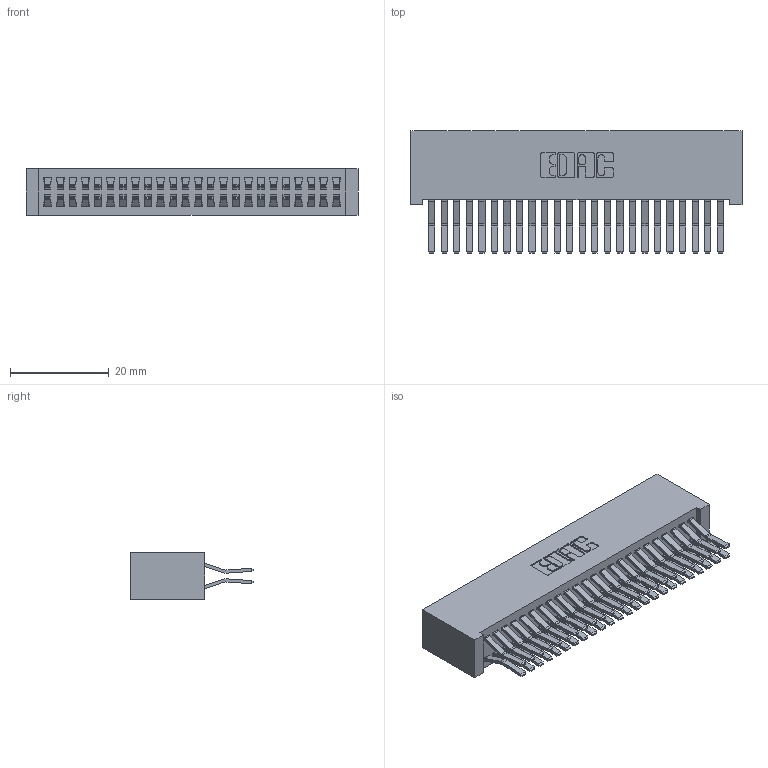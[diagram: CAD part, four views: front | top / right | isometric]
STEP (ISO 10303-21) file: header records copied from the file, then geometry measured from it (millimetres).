
FILE_DESCRIPTION (( 'STEP AP203' ), '1' );
FILE_NAME ('392-048-560-201.STEP', '2019-10-08T01:37:07', ( '' ), ( '' ), 'SwSTEP 2.0', 'SolidWorks 2016', '' );
FILE_SCHEMA (( 'CONFIG_CONTROL_DESIGN' ));
Length unit declared in the file: inch
Products named in the file (3): 342 Part_Lugless; 345-292-001_560 Tail; 392-048-560-201
Assembly tree (49 placements, depth 2):
  392-048-560-201
    342 Part_Lugless
    345-292-001_560 Tail  x48
Bounding box: 67.21 x 24.78 x 9.4 mm (x, y, z)
Volume: 6708.1 mm3; surface area: 11677.5 mm2
Topology: 49 solids, 49 shells, 2694 faces, 8003 edges, 5270 vertices
Faces by surface type: plane 1790, cylinder 904
Entity records: 17447 total; most frequent: CARTESIAN_POINT 2910, ORIENTED_EDGE 2846, DIRECTION 2515, EDGE_CURVE 1423, VECTOR 1299, LINE 1299, VERTEX_POINT 946, AXIS2_PLACEMENT_3D 608
